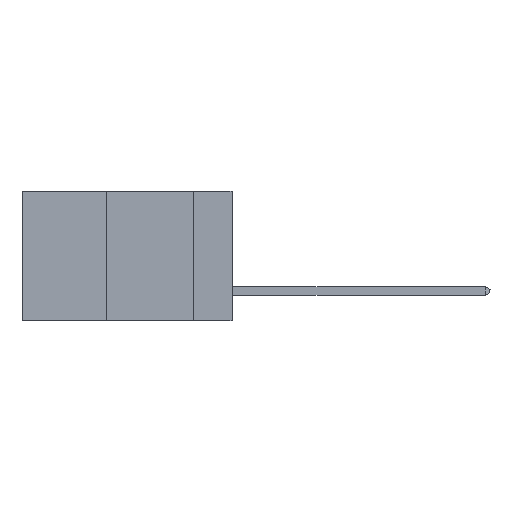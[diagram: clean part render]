
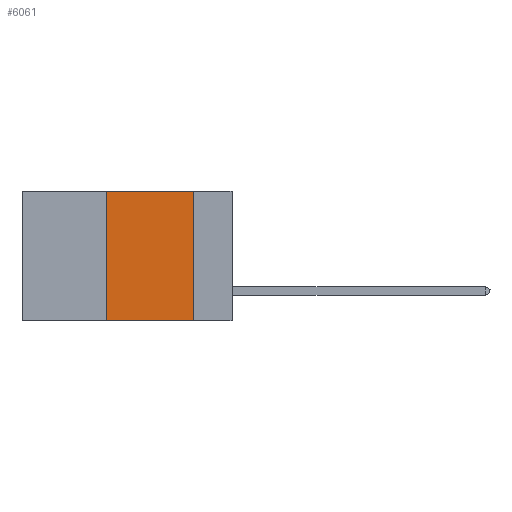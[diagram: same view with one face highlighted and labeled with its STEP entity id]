
A CAD part, left-side view. The second image highlights one B-rep face of the part: STEP entity #6061.
In plain terms, the highlighted planar face has unit normal (-1, 0, 0).
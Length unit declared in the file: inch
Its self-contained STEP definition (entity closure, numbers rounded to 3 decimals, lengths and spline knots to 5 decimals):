
#720 = VECTOR ( 'NONE', #8659, 39.37008 ) ;
#1089 = VECTOR ( 'NONE', #8877, 39.37008 ) ;
#2279 = LINE ( 'NONE', #6871, #1089 ) ;
#3580 = LINE ( 'NONE', #16097, #14721 ) ;
#5055 = ORIENTED_EDGE ( 'NONE', *, *, #13477, .F. ) ;
#5094 = ORIENTED_EDGE ( 'NONE', *, *, #20148, .F. ) ;
#5385 = LINE ( 'NONE', #20208, #720 ) ;
#6061 = ADVANCED_FACE ( 'NONE', ( #16533 ), #19147, .F. ) ;
#6620 = CARTESIAN_POINT ( 'NONE',  ( 0., 0.36, 0. ) ) ;
#6627 = VERTEX_POINT ( 'NONE', #18906 ) ;
#6871 = CARTESIAN_POINT ( 'NONE',  ( 0., 0.6, 0. ) ) ;
#7492 = CARTESIAN_POINT ( 'NONE',  ( 0., 0.36, -0.37 ) ) ;
#8208 = VECTOR ( 'NONE', #16780, 39.37008 ) ;
#8659 = DIRECTION ( 'NONE',  ( 0., -1., 0. ) ) ;
#8877 = DIRECTION ( 'NONE',  ( 0., -1., 0. ) ) ;
#9863 = ORIENTED_EDGE ( 'NONE', *, *, #19527, .T. ) ;
#11038 = AXIS2_PLACEMENT_3D ( 'NONE', #13638, #15167, #17126 ) ;
#12238 = VERTEX_POINT ( 'NONE', #17408 ) ;
#13477 = EDGE_CURVE ( 'NONE', #6627, #12238, #14193, .T. ) ;
#13638 = CARTESIAN_POINT ( 'NONE',  ( 0., 0.6, 0. ) ) ;
#14193 = LINE ( 'NONE', #24698, #8208 ) ;
#14721 = VECTOR ( 'NONE', #22164, 39.37008 ) ;
#15067 = EDGE_CURVE ( 'NONE', #17519, #20143, #3580, .T. ) ;
#15167 = DIRECTION ( 'NONE',  ( 1., 0., 0. ) ) ;
#16097 = CARTESIAN_POINT ( 'NONE',  ( 0., 0.36, 0. ) ) ;
#16533 = FACE_OUTER_BOUND ( 'NONE', #23966, .T. ) ;
#16780 = DIRECTION ( 'NONE',  ( 0., 0., -1. ) ) ;
#17126 = DIRECTION ( 'NONE',  ( 0., 0., -1. ) ) ;
#17408 = CARTESIAN_POINT ( 'NONE',  ( 0., 0.11, -0.37 ) ) ;
#17519 = VERTEX_POINT ( 'NONE', #7492 ) ;
#18906 = CARTESIAN_POINT ( 'NONE',  ( 0., 0.11, 0. ) ) ;
#19147 = PLANE ( 'NONE',  #11038 ) ;
#19527 = EDGE_CURVE ( 'NONE', #17519, #12238, #5385, .T. ) ;
#20143 = VERTEX_POINT ( 'NONE', #6620 ) ;
#20148 = EDGE_CURVE ( 'NONE', #20143, #6627, #2279, .T. ) ;
#20208 = CARTESIAN_POINT ( 'NONE',  ( 0., 0.6, -0.37 ) ) ;
#20905 = ORIENTED_EDGE ( 'NONE', *, *, #15067, .F. ) ;
#22164 = DIRECTION ( 'NONE',  ( 0., 0., 1. ) ) ;
#23966 = EDGE_LOOP ( 'NONE', ( #5055, #5094, #20905, #9863 ) ) ;
#24698 = CARTESIAN_POINT ( 'NONE',  ( 0., 0.11, 0. ) ) ;
